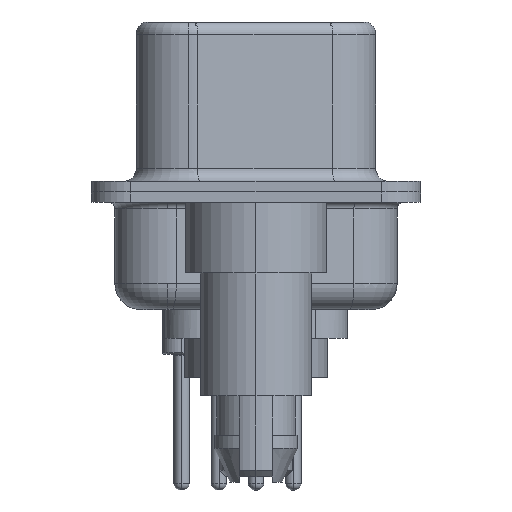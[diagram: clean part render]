
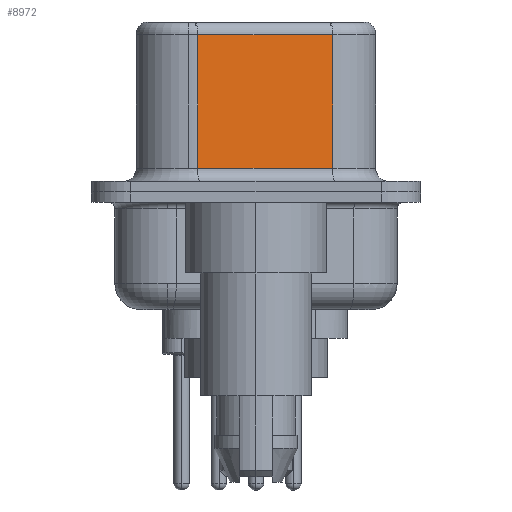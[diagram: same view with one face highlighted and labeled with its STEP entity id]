
A CAD part, left-side view. The second image highlights one B-rep face of the part: STEP entity #8972.
In plain terms, the highlighted planar face has unit normal (-0.985, -0.174, 0).
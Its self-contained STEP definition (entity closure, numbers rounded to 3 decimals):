
#76 = DIRECTION ( 'NONE',  ( 0., 0., -1. ) ) ;
#592 = ORIENTED_EDGE ( 'NONE', *, *, #15639, .F. ) ;
#953 = LINE ( 'NONE', #25017, #9992 ) ;
#1682 = CARTESIAN_POINT ( 'NONE',  ( 4.58, -2.927, 0.9 ) ) ;
#1971 = VECTOR ( 'NONE', #17226, 1000. ) ;
#2882 = ORIENTED_EDGE ( 'NONE', *, *, #21020, .T. ) ;
#4729 = PLANE ( 'NONE',  #10924 ) ;
#5021 = LINE ( 'NONE', #13599, #14765 ) ;
#6622 = DIRECTION ( 'NONE',  ( -0.174, 0.985, 0. ) ) ;
#8972 = ADVANCED_FACE ( 'NONE', ( #17096 ), #4729, .F. ) ;
#9137 = DIRECTION ( 'NONE',  ( 0., 0., -1. ) ) ;
#9992 = VECTOR ( 'NONE', #15061, 1000. ) ;
#10687 = ORIENTED_EDGE ( 'NONE', *, *, #19736, .T. ) ;
#10924 = AXIS2_PLACEMENT_3D ( 'NONE', #14405, #20351, #6622 ) ;
#10946 = VECTOR ( 'NONE', #9137, 1000. ) ;
#12844 = LINE ( 'NONE', #1682, #1971 ) ;
#13599 = CARTESIAN_POINT ( 'NONE',  ( 3.67, 2.233, 6.52 ) ) ;
#14148 = VERTEX_POINT ( 'NONE', #16507 ) ;
#14405 = CARTESIAN_POINT ( 'NONE',  ( 4.58, -2.927, 6.52 ) ) ;
#14423 = VERTEX_POINT ( 'NONE', #19217 ) ;
#14765 = VECTOR ( 'NONE', #76, 1000. ) ;
#15061 = DIRECTION ( 'NONE',  ( -0.174, 0.985, 0. ) ) ;
#15639 = EDGE_CURVE ( 'NONE', #14148, #24365, #21477, .T. ) ;
#15808 = ORIENTED_EDGE ( 'NONE', *, *, #16593, .T. ) ;
#16507 = CARTESIAN_POINT ( 'NONE',  ( 4.58, -2.927, 6.02 ) ) ;
#16593 = EDGE_CURVE ( 'NONE', #14148, #21685, #953, .T. ) ;
#17096 = FACE_OUTER_BOUND ( 'NONE', #19237, .T. ) ;
#17187 = CARTESIAN_POINT ( 'NONE',  ( 3.67, 2.233, 6.02 ) ) ;
#17226 = DIRECTION ( 'NONE',  ( 0.174, -0.985, 0. ) ) ;
#19217 = CARTESIAN_POINT ( 'NONE',  ( 3.67, 2.233, 0.9 ) ) ;
#19237 = EDGE_LOOP ( 'NONE', ( #592, #15808, #10687, #2882 ) ) ;
#19278 = CARTESIAN_POINT ( 'NONE',  ( 4.58, -2.927, 0.9 ) ) ;
#19736 = EDGE_CURVE ( 'NONE', #21685, #14423, #5021, .T. ) ;
#20351 = DIRECTION ( 'NONE',  ( 0.985, 0.174, 0. ) ) ;
#20973 = CARTESIAN_POINT ( 'NONE',  ( 4.58, -2.927, 6.52 ) ) ;
#21020 = EDGE_CURVE ( 'NONE', #14423, #24365, #12844, .T. ) ;
#21477 = LINE ( 'NONE', #20973, #10946 ) ;
#21685 = VERTEX_POINT ( 'NONE', #17187 ) ;
#24365 = VERTEX_POINT ( 'NONE', #19278 ) ;
#25017 = CARTESIAN_POINT ( 'NONE',  ( 4.58, -2.927, 6.02 ) ) ;
